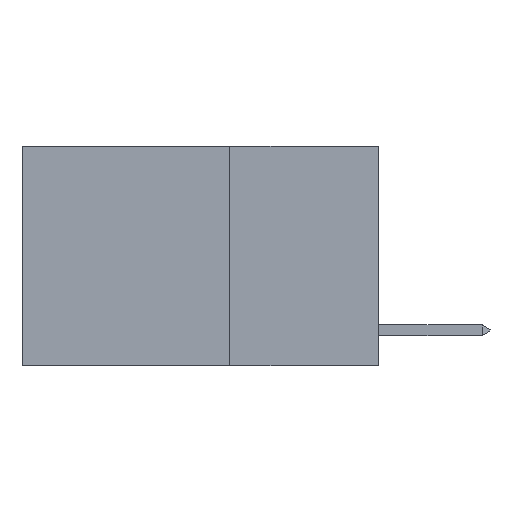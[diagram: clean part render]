
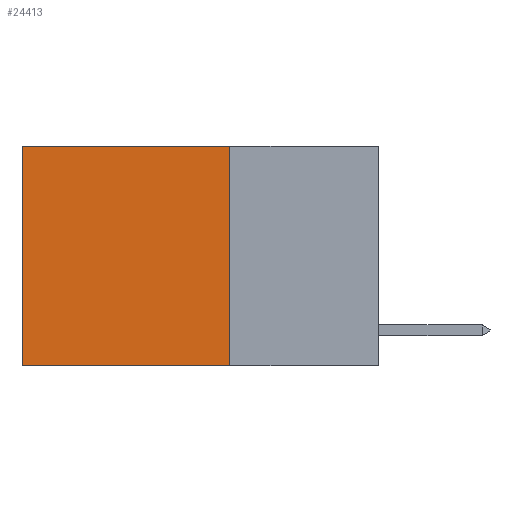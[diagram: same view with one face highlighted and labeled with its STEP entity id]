
A CAD part, left-side view. The second image highlights one B-rep face of the part: STEP entity #24413.
In plain terms, the highlighted planar face has unit normal (-1, 0, 0).
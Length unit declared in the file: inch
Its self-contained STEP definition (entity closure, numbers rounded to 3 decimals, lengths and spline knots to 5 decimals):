
#688 = CARTESIAN_POINT ( 'NONE',  ( 0.2625, 0.25, 0. ) ) ;
#2634 = EDGE_LOOP ( 'NONE', ( #10947, #15348, #14583, #8800 ) ) ;
#2786 = LINE ( 'NONE', #9744, #14495 ) ;
#4705 = PLANE ( 'NONE',  #5838 ) ;
#5806 = CARTESIAN_POINT ( 'NONE',  ( 0.2625, 0.6, 0. ) ) ;
#5838 = AXIS2_PLACEMENT_3D ( 'NONE', #13993, #21048, #7082 ) ;
#6371 = LINE ( 'NONE', #9365, #23593 ) ;
#7082 = DIRECTION ( 'NONE',  ( 0., 0., -1. ) ) ;
#8501 = FACE_OUTER_BOUND ( 'NONE', #2634, .T. ) ;
#8800 = ORIENTED_EDGE ( 'NONE', *, *, #21971, .T. ) ;
#9232 = DIRECTION ( 'NONE',  ( 0., 1., 0. ) ) ;
#9365 = CARTESIAN_POINT ( 'NONE',  ( 0.2625, 0.25, 0. ) ) ;
#9744 = CARTESIAN_POINT ( 'NONE',  ( 0.2625, 0.25, 0. ) ) ;
#10947 = ORIENTED_EDGE ( 'NONE', *, *, #17833, .T. ) ;
#11575 = CARTESIAN_POINT ( 'NONE',  ( 0.2625, 0.25, -0.37 ) ) ;
#11713 = DIRECTION ( 'NONE',  ( 0., 0., -1. ) ) ;
#13993 = CARTESIAN_POINT ( 'NONE',  ( 0.2625, 0.25, 0. ) ) ;
#14276 = VERTEX_POINT ( 'NONE', #21635 ) ;
#14495 = VECTOR ( 'NONE', #16807, 39.37008 ) ;
#14583 = ORIENTED_EDGE ( 'NONE', *, *, #23219, .F. ) ;
#15348 = ORIENTED_EDGE ( 'NONE', *, *, #27549, .F. ) ;
#15903 = LINE ( 'NONE', #16021, #22123 ) ;
#16021 = CARTESIAN_POINT ( 'NONE',  ( 0.2625, 0.6, 0. ) ) ;
#16192 = LINE ( 'NONE', #20884, #27929 ) ;
#16807 = DIRECTION ( 'NONE',  ( 0., 1., 0. ) ) ;
#17833 = EDGE_CURVE ( 'NONE', #22845, #14276, #15903, .T. ) ;
#20884 = CARTESIAN_POINT ( 'NONE',  ( 0.2625, 0.25, -0.37 ) ) ;
#21048 = DIRECTION ( 'NONE',  ( 1., 0., 0. ) ) ;
#21635 = CARTESIAN_POINT ( 'NONE',  ( 0.2625, 0.6, -0.37 ) ) ;
#21971 = EDGE_CURVE ( 'NONE', #23417, #22845, #2786, .T. ) ;
#22123 = VECTOR ( 'NONE', #23083, 39.37008 ) ;
#22845 = VERTEX_POINT ( 'NONE', #5806 ) ;
#23083 = DIRECTION ( 'NONE',  ( 0., 0., -1. ) ) ;
#23219 = EDGE_CURVE ( 'NONE', #23417, #27560, #6371, .T. ) ;
#23417 = VERTEX_POINT ( 'NONE', #688 ) ;
#23593 = VECTOR ( 'NONE', #11713, 39.37008 ) ;
#24413 = ADVANCED_FACE ( 'NONE', ( #8501 ), #4705, .F. ) ;
#27549 = EDGE_CURVE ( 'NONE', #27560, #14276, #16192, .T. ) ;
#27560 = VERTEX_POINT ( 'NONE', #11575 ) ;
#27929 = VECTOR ( 'NONE', #9232, 39.37008 ) ;
